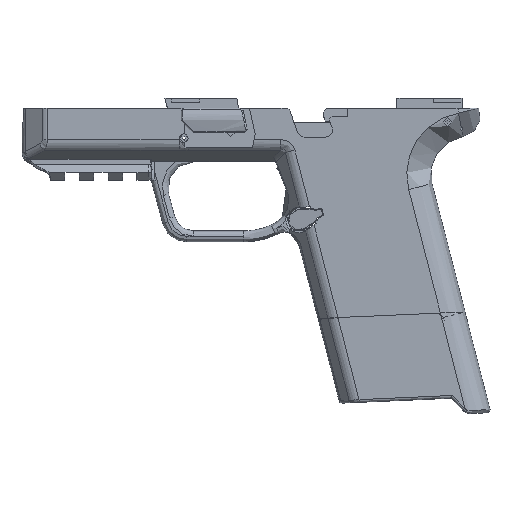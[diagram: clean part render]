
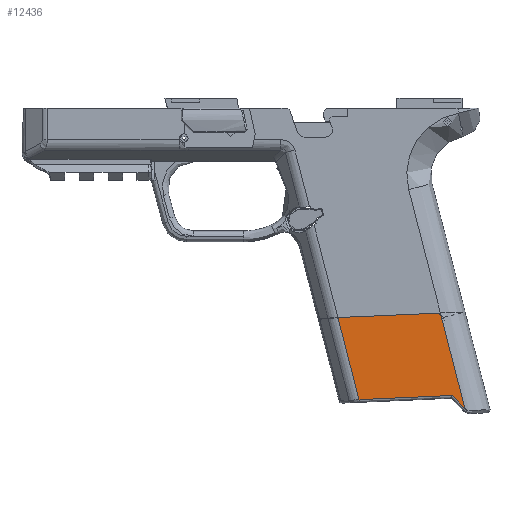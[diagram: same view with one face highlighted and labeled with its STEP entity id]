
A CAD part, left-side view. The second image highlights one B-rep face of the part: STEP entity #12436.
In plain terms, the highlighted face is planar.
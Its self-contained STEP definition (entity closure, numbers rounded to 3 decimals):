
#968=PLANE('',#13642);
#1626=FACE_OUTER_BOUND('',#2332,.T.);
#2332=EDGE_LOOP('',(#11433,#11434,#11435,#11436,#11437));
#3429=LINE('',#24108,#4559);
#3436=LINE('',#24229,#4566);
#3448=LINE('',#24260,#4578);
#3449=LINE('',#24264,#4579);
#3450=LINE('',#24265,#4580);
#4559=VECTOR('',#16833,10.);
#4566=VECTOR('',#16880,10.);
#4578=VECTOR('',#16914,10.);
#4579=VECTOR('',#16919,10.);
#4580=VECTOR('',#16920,10.);
#6044=VERTEX_POINT('',#23940);
#6055=VERTEX_POINT('',#24107);
#6069=VERTEX_POINT('',#24224);
#6077=VERTEX_POINT('',#24259);
#6078=VERTEX_POINT('',#24263);
#7839=EDGE_CURVE('',#6044,#6055,#3429,.T.);
#7862=EDGE_CURVE('',#6055,#6069,#3436,.T.);
#7877=EDGE_CURVE('',#6077,#6069,#3448,.T.);
#7879=EDGE_CURVE('',#6078,#6044,#3449,.T.);
#7880=EDGE_CURVE('',#6078,#6077,#3450,.T.);
#11433=ORIENTED_EDGE('',*,*,#7862,.F.);
#11434=ORIENTED_EDGE('',*,*,#7839,.F.);
#11435=ORIENTED_EDGE('',*,*,#7879,.F.);
#11436=ORIENTED_EDGE('',*,*,#7880,.T.);
#11437=ORIENTED_EDGE('',*,*,#7877,.T.);
#12436=ADVANCED_FACE('',(#1626),#968,.T.);
#13642=AXIS2_PLACEMENT_3D('',#24262,#16917,#16918);
#16833=DIRECTION('',(0.,0.697,-0.717));
#16880=DIRECTION('',(0.,0.999,0.044));
#16914=DIRECTION('',(0.,-0.249,0.969));
#16917=DIRECTION('center_axis',(1.,0.,0.));
#16918=DIRECTION('ref_axis',(0.,0.999,0.044));
#16919=DIRECTION('',(0.,-0.249,0.969));
#16920=DIRECTION('',(0.,0.999,0.044));
#23940=CARTESIAN_POINT('',(22.175,-83.635,101.607));
#24107=CARTESIAN_POINT('',(22.175,-79.055,96.902));
#24108=CARTESIAN_POINT('',(22.175,-73.411,91.103));
#24224=CARTESIAN_POINT('',(22.175,-45.112,98.406));
#24229=CARTESIAN_POINT('',(22.175,-44.983,98.411));
#24259=CARTESIAN_POINT('',(22.175,-37.447,68.587));
#24260=CARTESIAN_POINT('',(22.175,-37.447,68.587));
#24262=CARTESIAN_POINT('Origin',(22.175,-74.722,66.935));
#24263=CARTESIAN_POINT('',(22.175,-74.722,66.935));
#24264=CARTESIAN_POINT('',(22.175,-74.722,66.935));
#24265=CARTESIAN_POINT('',(22.175,-40.785,68.439));
